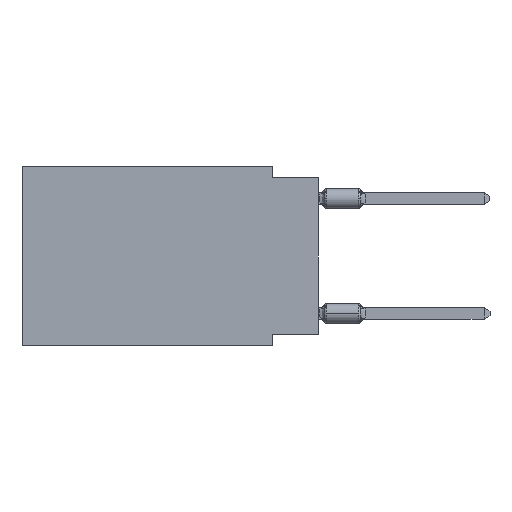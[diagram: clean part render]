
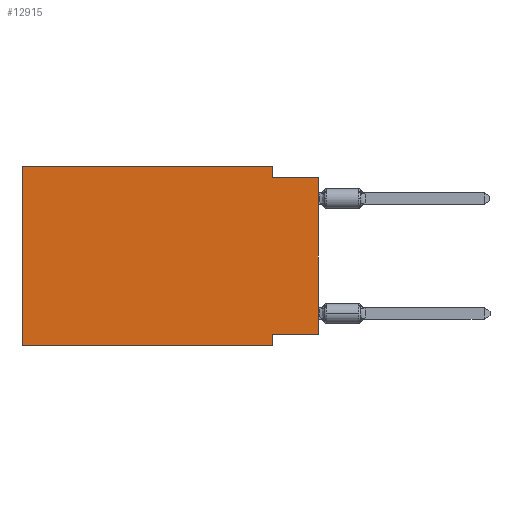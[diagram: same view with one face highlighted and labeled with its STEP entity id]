
A CAD part, left-side view. The second image highlights one B-rep face of the part: STEP entity #12915.
In plain terms, the highlighted planar face has unit normal (-1, 0, 0).
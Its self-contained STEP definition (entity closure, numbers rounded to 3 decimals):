
#226 = PLANE ( 'NONE',  #1933 ) ;
#594 = VERTEX_POINT ( 'NONE', #3861 ) ;
#679 = EDGE_CURVE ( 'NONE', #594, #4186, #1866, .T. ) ;
#877 = VERTEX_POINT ( 'NONE', #16708 ) ;
#1267 = CARTESIAN_POINT ( 'NONE',  ( 0., 16.383, -9.906 ) ) ;
#1615 = CARTESIAN_POINT ( 'NONE',  ( 0., 16.383, 0. ) ) ;
#1761 = EDGE_CURVE ( 'NONE', #5622, #15276, #7312, .T. ) ;
#1866 = LINE ( 'NONE', #14802, #4577 ) ;
#1933 = AXIS2_PLACEMENT_3D ( 'NONE', #1615, #9588, #2933 ) ;
#2559 = CARTESIAN_POINT ( 'NONE',  ( 0., 0., -9.271 ) ) ;
#2733 = LINE ( 'NONE', #13089, #13656 ) ;
#2924 = EDGE_CURVE ( 'NONE', #4186, #15276, #9490, .T. ) ;
#2925 = CARTESIAN_POINT ( 'NONE',  ( 0., 0., -0.635 ) ) ;
#2933 = DIRECTION ( 'NONE',  ( 0., 0., -1. ) ) ;
#3019 = DIRECTION ( 'NONE',  ( 0., -1., 0. ) ) ;
#3228 = CARTESIAN_POINT ( 'NONE',  ( 0., 0., -0.635 ) ) ;
#3371 = CARTESIAN_POINT ( 'NONE',  ( 0., 0., -9.271 ) ) ;
#3576 = VERTEX_POINT ( 'NONE', #16338 ) ;
#3787 = LINE ( 'NONE', #1267, #11782 ) ;
#3861 = CARTESIAN_POINT ( 'NONE',  ( 0., 2.54, 0. ) ) ;
#4037 = EDGE_CURVE ( 'NONE', #16007, #3576, #3787, .T. ) ;
#4112 = DIRECTION ( 'NONE',  ( 0., -1., 0. ) ) ;
#4186 = VERTEX_POINT ( 'NONE', #6633 ) ;
#4577 = VECTOR ( 'NONE', #7064, 1000. ) ;
#5231 = DIRECTION ( 'NONE',  ( 0., 1., 0. ) ) ;
#5519 = ORIENTED_EDGE ( 'NONE', *, *, #2924, .F. ) ;
#5622 = VERTEX_POINT ( 'NONE', #3371 ) ;
#6149 = ORIENTED_EDGE ( 'NONE', *, *, #1761, .T. ) ;
#6373 = LINE ( 'NONE', #2559, #16297 ) ;
#6633 = CARTESIAN_POINT ( 'NONE',  ( 0., 2.54, -0.635 ) ) ;
#6685 = VECTOR ( 'NONE', #3019, 1000. ) ;
#6986 = FACE_OUTER_BOUND ( 'NONE', #9815, .T. ) ;
#7064 = DIRECTION ( 'NONE',  ( 0., 0., -1. ) ) ;
#7312 = LINE ( 'NONE', #12455, #9822 ) ;
#7357 = EDGE_CURVE ( 'NONE', #877, #594, #12222, .T. ) ;
#7621 = EDGE_CURVE ( 'NONE', #8233, #3576, #2733, .T. ) ;
#8233 = VERTEX_POINT ( 'NONE', #10692 ) ;
#8432 = VECTOR ( 'NONE', #4112, 1000. ) ;
#8519 = ORIENTED_EDGE ( 'NONE', *, *, #15449, .F. ) ;
#8984 = DIRECTION ( 'NONE',  ( 0., 0., -1. ) ) ;
#9340 = ORIENTED_EDGE ( 'NONE', *, *, #7357, .F. ) ;
#9490 = LINE ( 'NONE', #2925, #8432 ) ;
#9588 = DIRECTION ( 'NONE',  ( 1., 0., 0. ) ) ;
#9815 = EDGE_LOOP ( 'NONE', ( #6149, #5519, #15016, #9340, #8519, #12130, #11014, #13902 ) ) ;
#9822 = VECTOR ( 'NONE', #11231, 1000. ) ;
#10692 = CARTESIAN_POINT ( 'NONE',  ( 0., 2.54, -9.271 ) ) ;
#10750 = LINE ( 'NONE', #13289, #11081 ) ;
#11014 = ORIENTED_EDGE ( 'NONE', *, *, #7621, .F. ) ;
#11081 = VECTOR ( 'NONE', #15801, 1000. ) ;
#11231 = DIRECTION ( 'NONE',  ( 0., 0., 1. ) ) ;
#11235 = CARTESIAN_POINT ( 'NONE',  ( 0., 16.383, -9.906 ) ) ;
#11538 = DIRECTION ( 'NONE',  ( 0., -1., 0. ) ) ;
#11782 = VECTOR ( 'NONE', #11538, 1000. ) ;
#11857 = EDGE_CURVE ( 'NONE', #5622, #8233, #6373, .T. ) ;
#12130 = ORIENTED_EDGE ( 'NONE', *, *, #4037, .T. ) ;
#12222 = LINE ( 'NONE', #16290, #6685 ) ;
#12455 = CARTESIAN_POINT ( 'NONE',  ( 0., 0., 0. ) ) ;
#12915 = ADVANCED_FACE ( 'NONE', ( #6986 ), #226, .F. ) ;
#13089 = CARTESIAN_POINT ( 'NONE',  ( 0., 2.54, -9.906 ) ) ;
#13289 = CARTESIAN_POINT ( 'NONE',  ( 0., 16.383, 0. ) ) ;
#13656 = VECTOR ( 'NONE', #8984, 1000. ) ;
#13902 = ORIENTED_EDGE ( 'NONE', *, *, #11857, .F. ) ;
#14802 = CARTESIAN_POINT ( 'NONE',  ( 0., 2.54, 0. ) ) ;
#15016 = ORIENTED_EDGE ( 'NONE', *, *, #679, .F. ) ;
#15276 = VERTEX_POINT ( 'NONE', #3228 ) ;
#15449 = EDGE_CURVE ( 'NONE', #16007, #877, #10750, .T. ) ;
#15801 = DIRECTION ( 'NONE',  ( 0., 0., 1. ) ) ;
#16007 = VERTEX_POINT ( 'NONE', #11235 ) ;
#16290 = CARTESIAN_POINT ( 'NONE',  ( 0., 16.383, 0. ) ) ;
#16297 = VECTOR ( 'NONE', #5231, 1000. ) ;
#16338 = CARTESIAN_POINT ( 'NONE',  ( 0., 2.54, -9.906 ) ) ;
#16708 = CARTESIAN_POINT ( 'NONE',  ( 0., 16.383, 0. ) ) ;
